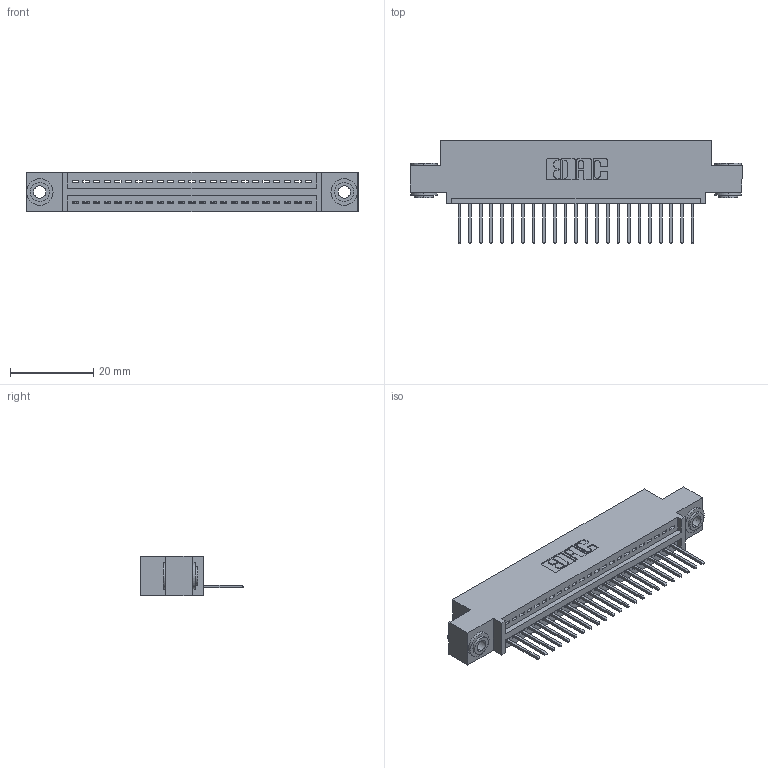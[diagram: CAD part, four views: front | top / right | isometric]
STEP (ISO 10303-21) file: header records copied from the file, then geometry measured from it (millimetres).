
FILE_DESCRIPTION (( 'STEP AP203' ), '1' );
FILE_NAME ('395-023-523-403.STEP', '2018-11-08T07:54:34', ( '' ), ( '' ), 'SwSTEP 2.0', 'SolidWorks 2016', '' );
FILE_SCHEMA (( 'CONFIG_CONTROL_DESIGN' ));
Length unit declared in the file: inch
Products named in the file (4): 345-250-002_345-250-002-102; 345 Part_0.110 Offset - 0.156 Dia-TH; 345-292-001_345-293-123; 395-023-523-403
Assembly tree (26 placements, depth 2):
  395-023-523-403
    345 Part_0.110 Offset - 0.156 Dia-TH
    345-292-001_345-293-123  x23
    345-250-002_345-250-002-102  x2
Bounding box: 79.63 x 24.82 x 9.4 mm (x, y, z)
Volume: 7344.7 mm3; surface area: 9823.7 mm2
Topology: 26 solids, 26 shells, 1502 faces, 4477 edges, 2950 vertices
Faces by surface type: plane 1014, cylinder 480, cone 8
Entity records: 20668 total; most frequent: CARTESIAN_POINT 3560, ORIENTED_EDGE 3510, DIRECTION 3167, EDGE_CURVE 1755, LINE 1507, VECTOR 1507, VERTEX_POINT 1166, AXIS2_PLACEMENT_3D 830
